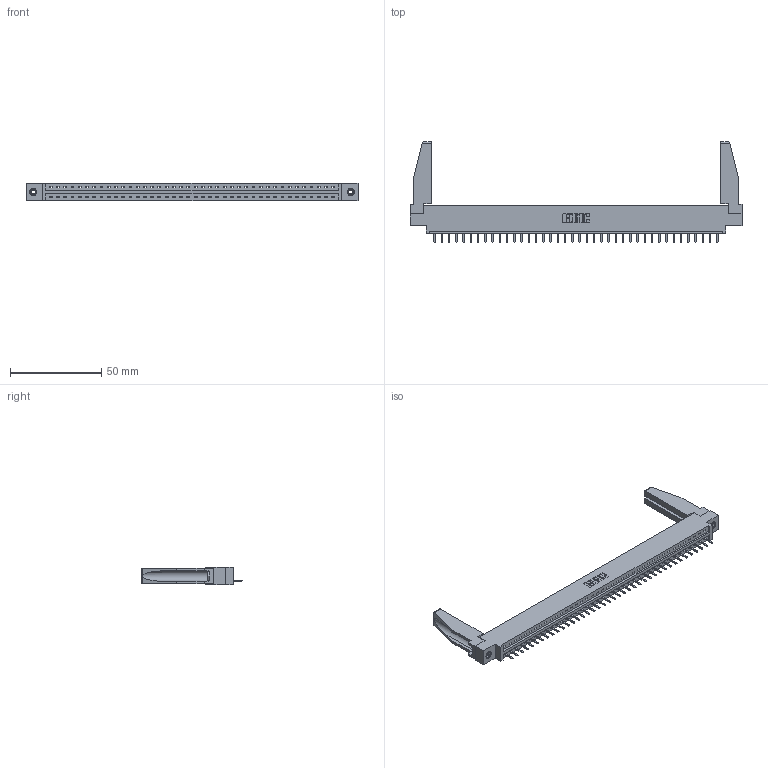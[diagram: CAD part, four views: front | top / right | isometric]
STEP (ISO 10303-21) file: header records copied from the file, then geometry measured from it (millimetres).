
FILE_DESCRIPTION (( 'STEP AP203' ), '1' );
FILE_NAME ('387-040-520-678.STEP', '2019-10-04T18:22:23', ( '' ), ( '' ), 'SwSTEP 2.0', 'SolidWorks 2016', '' );
FILE_SCHEMA (( 'CONFIG_CONTROL_DESIGN' ));
Length unit declared in the file: inch
Products named in the file (5): 307-220-078; 345-250-001_345-250-001-102; 337 Part_0.170 Offset - 0.156 Dia-TI; 387-040-520-678; 345-292-001_345-293-120
Assembly tree (45 placements, depth 2):
  387-040-520-678
    337 Part_0.170 Offset - 0.156 Dia-TI
    345-292-001_345-293-120  x40
    345-250-001_345-250-001-102  x2
    307-220-078  x2
Bounding box: 181.51 x 54.82 x 9.4 mm (x, y, z)
Volume: 22600.5 mm3; surface area: 22735.8 mm2
Topology: 45 solids, 45 shells, 2888 faces, 8493 edges, 5546 vertices
Faces by surface type: plane 2078, cylinder 794, cone 12, torus 4
Entity records: 32678 total; most frequent: CARTESIAN_POINT 5696, ORIENTED_EDGE 5616, DIRECTION 4796, EDGE_CURVE 2808, VECTOR 2638, LINE 2638, VERTEX_POINT 1864, AXIS2_PLACEMENT_3D 1079
